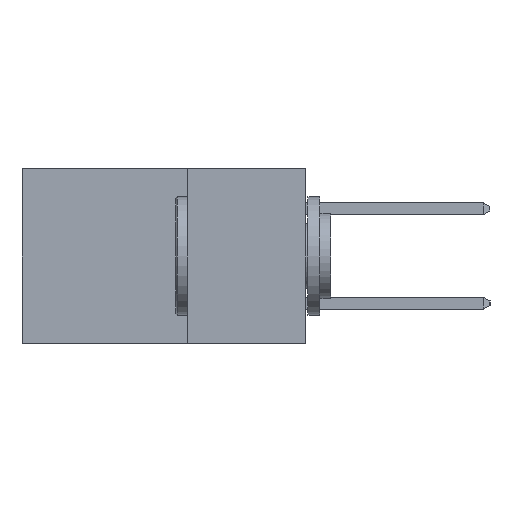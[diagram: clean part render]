
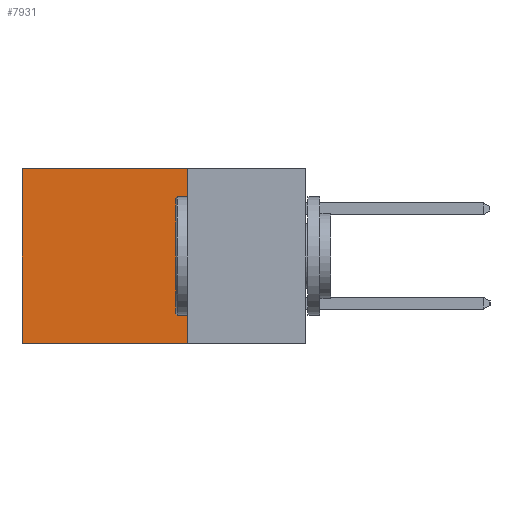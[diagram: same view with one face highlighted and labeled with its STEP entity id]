
A CAD part, left-side view. The second image highlights one B-rep face of the part: STEP entity #7931.
In plain terms, the highlighted planar face has unit normal (-1, 0, 0).
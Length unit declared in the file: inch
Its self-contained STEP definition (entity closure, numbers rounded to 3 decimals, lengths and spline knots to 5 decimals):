
#310 = VERTEX_POINT ( 'NONE', #11076 ) ;
#2831 = CARTESIAN_POINT ( 'NONE',  ( 0.2615, 0.25, -0.37 ) ) ;
#2899 = DIRECTION ( 'NONE',  ( 0., 0., -1. ) ) ;
#2990 = LINE ( 'NONE', #10687, #11128 ) ;
#4763 = VERTEX_POINT ( 'NONE', #13286 ) ;
#4797 = VECTOR ( 'NONE', #5110, 39.37008 ) ;
#5094 = CARTESIAN_POINT ( 'NONE',  ( 0.2615, 0.25, 0. ) ) ;
#5110 = DIRECTION ( 'NONE',  ( 0., 1., 0. ) ) ;
#5125 = LINE ( 'NONE', #5094, #4797 ) ;
#5461 = FACE_OUTER_BOUND ( 'NONE', #5561, .T. ) ;
#5499 = AXIS2_PLACEMENT_3D ( 'NONE', #12863, #12856, #12841 ) ;
#5561 = EDGE_LOOP ( 'NONE', ( #10340, #12784, #10025, #12013 ) ) ;
#6856 = CARTESIAN_POINT ( 'NONE',  ( 0.2615, 0.6, -0.37 ) ) ;
#6904 = LINE ( 'NONE', #6856, #12182 ) ;
#6926 = DIRECTION ( 'NONE',  ( 0., 0., -1. ) ) ;
#7189 = VERTEX_POINT ( 'NONE', #10445 ) ;
#7482 = EDGE_CURVE ( 'NONE', #4763, #8302, #5125, .T. ) ;
#7600 = EDGE_CURVE ( 'NONE', #4763, #7189, #9186, .T. ) ;
#7931 = ADVANCED_FACE ( 'NONE', ( #5461 ), #13105, .F. ) ;
#8302 = VERTEX_POINT ( 'NONE', #10944 ) ;
#8344 = EDGE_CURVE ( 'NONE', #7189, #310, #2990, .T. ) ;
#9186 = LINE ( 'NONE', #2831, #11971 ) ;
#10025 = ORIENTED_EDGE ( 'NONE', *, *, #7600, .F. ) ;
#10340 = ORIENTED_EDGE ( 'NONE', *, *, #11268, .T. ) ;
#10445 = CARTESIAN_POINT ( 'NONE',  ( 0.2615, 0.25, -0.37 ) ) ;
#10632 = DIRECTION ( 'NONE',  ( 0., 1., 0. ) ) ;
#10687 = CARTESIAN_POINT ( 'NONE',  ( 0.2615, 0.25, -0.37 ) ) ;
#10944 = CARTESIAN_POINT ( 'NONE',  ( 0.2615, 0.6, 0. ) ) ;
#11076 = CARTESIAN_POINT ( 'NONE',  ( 0.2615, 0.6, -0.37 ) ) ;
#11128 = VECTOR ( 'NONE', #10632, 39.37008 ) ;
#11268 = EDGE_CURVE ( 'NONE', #8302, #310, #6904, .T. ) ;
#11971 = VECTOR ( 'NONE', #2899, 39.37008 ) ;
#12013 = ORIENTED_EDGE ( 'NONE', *, *, #7482, .T. ) ;
#12182 = VECTOR ( 'NONE', #6926, 39.37008 ) ;
#12784 = ORIENTED_EDGE ( 'NONE', *, *, #8344, .F. ) ;
#12841 = DIRECTION ( 'NONE',  ( 0., 0., -1. ) ) ;
#12856 = DIRECTION ( 'NONE',  ( 1., 0., 0. ) ) ;
#12863 = CARTESIAN_POINT ( 'NONE',  ( 0.2615, 0.25, -0.37 ) ) ;
#13105 = PLANE ( 'NONE',  #5499 ) ;
#13286 = CARTESIAN_POINT ( 'NONE',  ( 0.2615, 0.25, 0. ) ) ;
